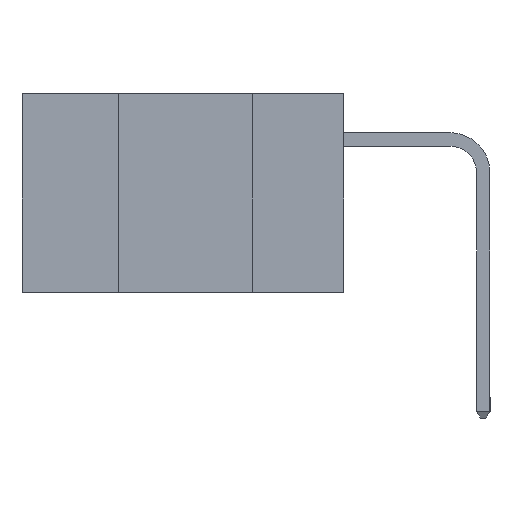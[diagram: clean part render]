
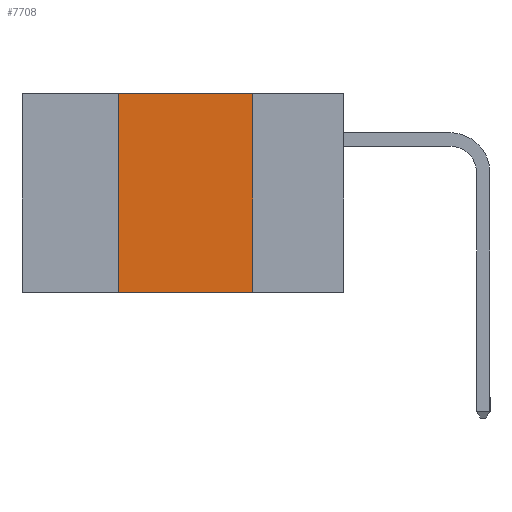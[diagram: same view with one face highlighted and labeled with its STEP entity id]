
A CAD part, left-side view. The second image highlights one B-rep face of the part: STEP entity #7708.
In plain terms, the highlighted planar face has unit normal (-1, 0, 0).
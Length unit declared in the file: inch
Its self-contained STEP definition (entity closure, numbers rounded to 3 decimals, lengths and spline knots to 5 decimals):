
#1001 = ORIENTED_EDGE ( 'NONE', *, *, #3842, .T. ) ;
#2308 = VECTOR ( 'NONE', #10560, 39.37008 ) ;
#3206 = DIRECTION ( 'NONE',  ( 0., 0., -1. ) ) ;
#3842 = EDGE_CURVE ( 'NONE', #16933, #8580, #21876, .T. ) ;
#4123 = LINE ( 'NONE', #12730, #18084 ) ;
#5118 = EDGE_CURVE ( 'NONE', #16933, #13543, #15763, .T. ) ;
#5616 = VECTOR ( 'NONE', #23521, 39.37008 ) ;
#6381 = EDGE_CURVE ( 'NONE', #13543, #10409, #7317, .T. ) ;
#7317 = LINE ( 'NONE', #10705, #2308 ) ;
#7708 = ADVANCED_FACE ( 'NONE', ( #17136 ), #11606, .F. ) ;
#8265 = EDGE_LOOP ( 'NONE', ( #13194, #8680, #9277, #1001 ) ) ;
#8580 = VERTEX_POINT ( 'NONE', #8872 ) ;
#8680 = ORIENTED_EDGE ( 'NONE', *, *, #6381, .F. ) ;
#8872 = CARTESIAN_POINT ( 'NONE',  ( 0., 0.17, -0.37 ) ) ;
#9277 = ORIENTED_EDGE ( 'NONE', *, *, #5118, .F. ) ;
#10232 = EDGE_CURVE ( 'NONE', #10409, #8580, #4123, .T. ) ;
#10409 = VERTEX_POINT ( 'NONE', #16936 ) ;
#10560 = DIRECTION ( 'NONE',  ( 0., -1., 0. ) ) ;
#10687 = DIRECTION ( 'NONE',  ( 0., -1., 0. ) ) ;
#10705 = CARTESIAN_POINT ( 'NONE',  ( 0., 0.6, 0. ) ) ;
#10765 = CARTESIAN_POINT ( 'NONE',  ( 0., 0.6, -0.37 ) ) ;
#10766 = VECTOR ( 'NONE', #10687, 39.37008 ) ;
#10994 = AXIS2_PLACEMENT_3D ( 'NONE', #11271, #11169, #11136 ) ;
#11136 = DIRECTION ( 'NONE',  ( 0., 0., -1. ) ) ;
#11169 = DIRECTION ( 'NONE',  ( 1., 0., 0. ) ) ;
#11271 = CARTESIAN_POINT ( 'NONE',  ( 0., 0.6, 0. ) ) ;
#11606 = PLANE ( 'NONE',  #10994 ) ;
#12205 = CARTESIAN_POINT ( 'NONE',  ( 0., 0.42, 0. ) ) ;
#12730 = CARTESIAN_POINT ( 'NONE',  ( 0., 0.17, -0.37 ) ) ;
#13194 = ORIENTED_EDGE ( 'NONE', *, *, #10232, .F. ) ;
#13543 = VERTEX_POINT ( 'NONE', #12205 ) ;
#15763 = LINE ( 'NONE', #23570, #5616 ) ;
#16933 = VERTEX_POINT ( 'NONE', #17531 ) ;
#16936 = CARTESIAN_POINT ( 'NONE',  ( 0., 0.17, 0. ) ) ;
#17136 = FACE_OUTER_BOUND ( 'NONE', #8265, .T. ) ;
#17531 = CARTESIAN_POINT ( 'NONE',  ( 0., 0.42, -0.37 ) ) ;
#18084 = VECTOR ( 'NONE', #3206, 39.37008 ) ;
#21876 = LINE ( 'NONE', #10765, #10766 ) ;
#23521 = DIRECTION ( 'NONE',  ( 0., 0., 1. ) ) ;
#23570 = CARTESIAN_POINT ( 'NONE',  ( 0., 0.42, -0.37 ) ) ;
